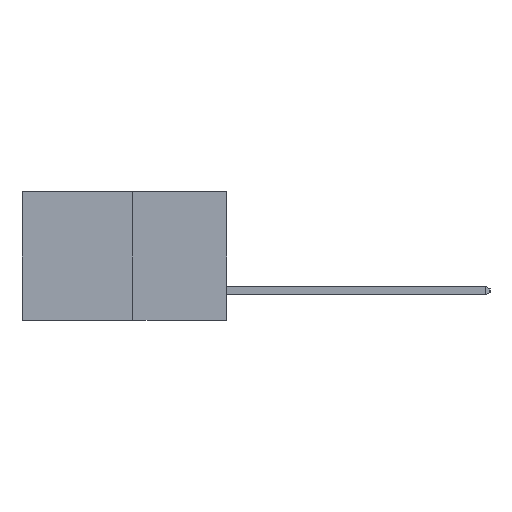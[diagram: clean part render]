
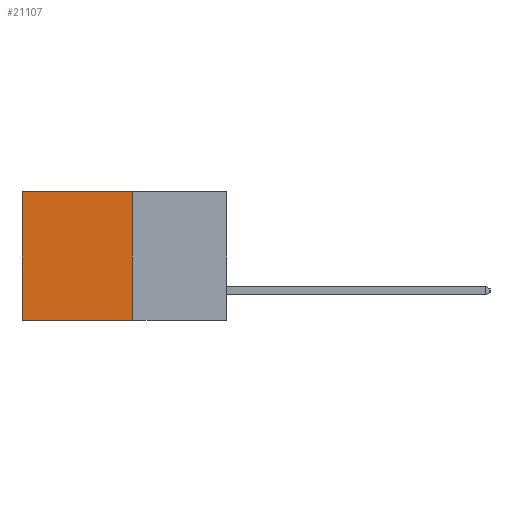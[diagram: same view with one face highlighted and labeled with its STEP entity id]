
A CAD part, left-side view. The second image highlights one B-rep face of the part: STEP entity #21107.
In plain terms, the highlighted planar face has unit normal (-1, 0, 0).
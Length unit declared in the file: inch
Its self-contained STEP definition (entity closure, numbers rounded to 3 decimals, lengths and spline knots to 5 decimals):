
#1455 = VECTOR ( 'NONE', #9190, 39.37008 ) ;
#1796 = CARTESIAN_POINT ( 'NONE',  ( 0.277, 0.27, 0. ) ) ;
#3725 = CARTESIAN_POINT ( 'NONE',  ( 0.277, 0.27, 0. ) ) ;
#4802 = CARTESIAN_POINT ( 'NONE',  ( 0.277, 0.27, -0.37 ) ) ;
#5003 = FACE_OUTER_BOUND ( 'NONE', #13119, .T. ) ;
#5222 = VERTEX_POINT ( 'NONE', #17965 ) ;
#5970 = EDGE_CURVE ( 'NONE', #16346, #11918, #17111, .T. ) ;
#6578 = VECTOR ( 'NONE', #19328, 39.37008 ) ;
#7783 = DIRECTION ( 'NONE',  ( 1., 0., 0. ) ) ;
#9190 = DIRECTION ( 'NONE',  ( 0., 0., -1. ) ) ;
#9863 = CARTESIAN_POINT ( 'NONE',  ( 0.277, 0.59, -0.37 ) ) ;
#10149 = ORIENTED_EDGE ( 'NONE', *, *, #14219, .F. ) ;
#10337 = VERTEX_POINT ( 'NONE', #1796 ) ;
#11674 = LINE ( 'NONE', #15934, #16213 ) ;
#11918 = VERTEX_POINT ( 'NONE', #9863 ) ;
#12645 = LINE ( 'NONE', #4802, #22153 ) ;
#12963 = ORIENTED_EDGE ( 'NONE', *, *, #23334, .F. ) ;
#13119 = EDGE_LOOP ( 'NONE', ( #21014, #10149, #12963, #24406 ) ) ;
#13170 = EDGE_CURVE ( 'NONE', #10337, #16346, #21918, .T. ) ;
#13556 = PLANE ( 'NONE',  #16663 ) ;
#14078 = DIRECTION ( 'NONE',  ( 0., 0., -1. ) ) ;
#14219 = EDGE_CURVE ( 'NONE', #5222, #11918, #12645, .T. ) ;
#14600 = DIRECTION ( 'NONE',  ( 0., 1., 0. ) ) ;
#15934 = CARTESIAN_POINT ( 'NONE',  ( 0.277, 0.27, -0.37 ) ) ;
#15998 = CARTESIAN_POINT ( 'NONE',  ( 0.277, 0.59, -0.37 ) ) ;
#16213 = VECTOR ( 'NONE', #14078, 39.37008 ) ;
#16346 = VERTEX_POINT ( 'NONE', #23727 ) ;
#16663 = AXIS2_PLACEMENT_3D ( 'NONE', #19345, #7783, #21210 ) ;
#17111 = LINE ( 'NONE', #15998, #1455 ) ;
#17965 = CARTESIAN_POINT ( 'NONE',  ( 0.277, 0.27, -0.37 ) ) ;
#19328 = DIRECTION ( 'NONE',  ( 0., 1., 0. ) ) ;
#19345 = CARTESIAN_POINT ( 'NONE',  ( 0.277, 0.27, -0.37 ) ) ;
#21014 = ORIENTED_EDGE ( 'NONE', *, *, #5970, .T. ) ;
#21107 = ADVANCED_FACE ( 'NONE', ( #5003 ), #13556, .F. ) ;
#21210 = DIRECTION ( 'NONE',  ( 0., 0., -1. ) ) ;
#21918 = LINE ( 'NONE', #3725, #6578 ) ;
#22153 = VECTOR ( 'NONE', #14600, 39.37008 ) ;
#23334 = EDGE_CURVE ( 'NONE', #10337, #5222, #11674, .T. ) ;
#23727 = CARTESIAN_POINT ( 'NONE',  ( 0.277, 0.59, 0. ) ) ;
#24406 = ORIENTED_EDGE ( 'NONE', *, *, #13170, .T. ) ;
